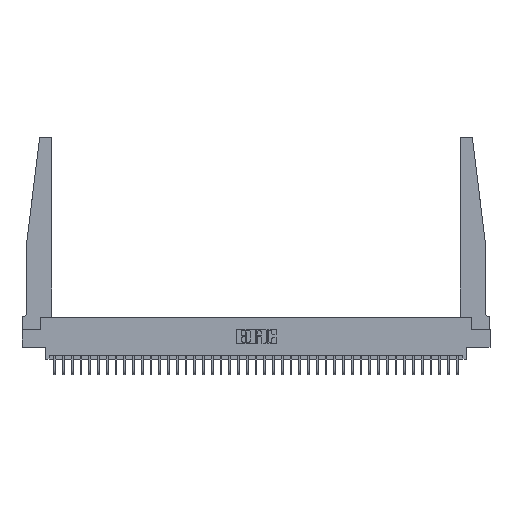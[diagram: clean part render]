
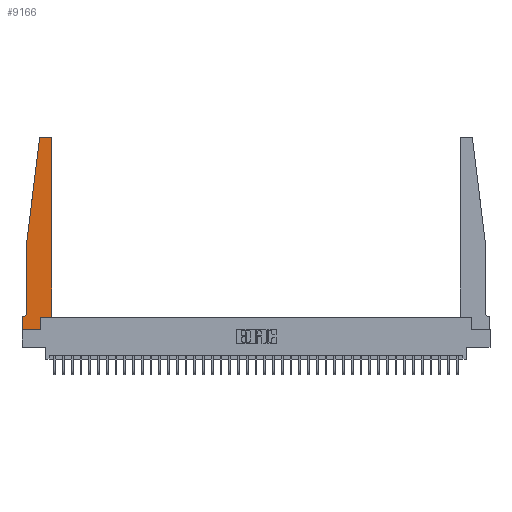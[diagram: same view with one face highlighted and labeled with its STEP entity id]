
A CAD part, top view. The second image highlights one B-rep face of the part: STEP entity #9166.
In plain terms, the highlighted planar face has unit normal (0, 0, 1).
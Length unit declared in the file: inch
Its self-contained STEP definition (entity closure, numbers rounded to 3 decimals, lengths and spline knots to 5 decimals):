
#387 = VERTEX_POINT ( 'NONE', #12092 ) ;
#510 = LINE ( 'NONE', #29118, #29665 ) ;
#821 = EDGE_CURVE ( 'NONE', #387, #16266, #21222, .T. ) ;
#1296 = DIRECTION ( 'NONE',  ( 0., 1., 0. ) ) ;
#1313 = EDGE_CURVE ( 'NONE', #24531, #387, #5923, .T. ) ;
#1544 = CARTESIAN_POINT ( 'NONE',  ( 0.25, 2.75, 0.37 ) ) ;
#2374 = VERTEX_POINT ( 'NONE', #12447 ) ;
#2948 = DIRECTION ( 'NONE',  ( -0.122, -0.992, 0. ) ) ;
#3323 = VECTOR ( 'NONE', #33705, 39.37008 ) ;
#3333 = CARTESIAN_POINT ( 'NONE',  ( 0.395, 2.72, 0.37 ) ) ;
#4560 = CARTESIAN_POINT ( 'NONE',  ( 0., 0., 0.37 ) ) ;
#5331 = ORIENTED_EDGE ( 'NONE', *, *, #36915, .T. ) ;
#5678 = VERTEX_POINT ( 'NONE', #19425 ) ;
#5923 = LINE ( 'NONE', #20399, #12283 ) ;
#6107 = CARTESIAN_POINT ( 'NONE',  ( 0.065, 1.25, 0.37 ) ) ;
#6130 = ORIENTED_EDGE ( 'NONE', *, *, #17333, .T. ) ;
#6385 = CARTESIAN_POINT ( 'NONE',  ( 0., 0., 0.37 ) ) ;
#6707 = ORIENTED_EDGE ( 'NONE', *, *, #17545, .T. ) ;
#7397 = ORIENTED_EDGE ( 'NONE', *, *, #15008, .T. ) ;
#8469 = LINE ( 'NONE', #19943, #34040 ) ;
#8623 = CARTESIAN_POINT ( 'NONE',  ( 0., 0., 0.37 ) ) ;
#8785 = DIRECTION ( 'NONE',  ( 1., 0., 0. ) ) ;
#9166 = ADVANCED_FACE ( 'NONE', ( #25499 ), #31516, .T. ) ;
#9380 = DIRECTION ( 'NONE',  ( 0., -1., 0. ) ) ;
#10082 = VERTEX_POINT ( 'NONE', #34422 ) ;
#10230 = EDGE_LOOP ( 'NONE', ( #35378, #15168, #11102, #34128, #7397, #25515, #29548, #6130, #5331, #6707, #31524, #20051 ) ) ;
#10434 = LINE ( 'NONE', #10616, #3323 ) ;
#10616 = CARTESIAN_POINT ( 'NONE',  ( 0.065, 0.1875, 0.37 ) ) ;
#11102 = ORIENTED_EDGE ( 'NONE', *, *, #15482, .T. ) ;
#11567 = CIRCLE ( 'NONE', #34339, 0.03 ) ;
#12092 = CARTESIAN_POINT ( 'NONE',  ( 0.425, 2.72, 0.37 ) ) ;
#12154 = CIRCLE ( 'NONE', #12748, 0.05 ) ;
#12283 = VECTOR ( 'NONE', #14789, 39.37008 ) ;
#12390 = DIRECTION ( 'NONE',  ( 0., 0., 1. ) ) ;
#12447 = CARTESIAN_POINT ( 'NONE',  ( 0.015, 0.1875, 0.37 ) ) ;
#12464 = VECTOR ( 'NONE', #35587, 39.37008 ) ;
#12748 = AXIS2_PLACEMENT_3D ( 'NONE', #20483, #17690, #29151 ) ;
#13088 = CARTESIAN_POINT ( 'NONE',  ( 0.27653, 2.75, 0.37 ) ) ;
#13323 = AXIS2_PLACEMENT_3D ( 'NONE', #28693, #31137, #14417 ) ;
#13412 = LINE ( 'NONE', #4560, #12464 ) ;
#14417 = DIRECTION ( 'NONE',  ( 1., 0., 0. ) ) ;
#14789 = DIRECTION ( 'NONE',  ( 0., 1., 0. ) ) ;
#14844 = DIRECTION ( 'NONE',  ( 0., -1., 0. ) ) ;
#15008 = EDGE_CURVE ( 'NONE', #25656, #2374, #12154, .T. ) ;
#15168 = ORIENTED_EDGE ( 'NONE', *, *, #31744, .T. ) ;
#15482 = EDGE_CURVE ( 'NONE', #10082, #15915, #34343, .T. ) ;
#15915 = VERTEX_POINT ( 'NONE', #6107 ) ;
#16266 = VERTEX_POINT ( 'NONE', #29349 ) ;
#16661 = CARTESIAN_POINT ( 'NONE',  ( 0., 0.1875, 0.37 ) ) ;
#16793 = DIRECTION ( 'NONE',  ( 1., 0., 0. ) ) ;
#17333 = EDGE_CURVE ( 'NONE', #31062, #22013, #13412, .T. ) ;
#17545 = EDGE_CURVE ( 'NONE', #5678, #24531, #8469, .T. ) ;
#17690 = DIRECTION ( 'NONE',  ( 0., 0., -1. ) ) ;
#18093 = EDGE_CURVE ( 'NONE', #36003, #31062, #25903, .T. ) ;
#19425 = CARTESIAN_POINT ( 'NONE',  ( 0.2605, 0.18, 0.37 ) ) ;
#19794 = CARTESIAN_POINT ( 'NONE',  ( 0.27653, 2.72, 0.37 ) ) ;
#19871 = CARTESIAN_POINT ( 'NONE',  ( 0.065, 0.2375, 0.37 ) ) ;
#19943 = CARTESIAN_POINT ( 'NONE',  ( 0.425, 0.18, 0.37 ) ) ;
#20051 = ORIENTED_EDGE ( 'NONE', *, *, #821, .T. ) ;
#20399 = CARTESIAN_POINT ( 'NONE',  ( 0.425, 0.18, 0.37 ) ) ;
#20483 = CARTESIAN_POINT ( 'NONE',  ( 0.015, 0.2375, 0.37 ) ) ;
#21222 = CIRCLE ( 'NONE', #33804, 0.03 ) ;
#22013 = VERTEX_POINT ( 'NONE', #32024 ) ;
#23125 = EDGE_CURVE ( 'NONE', #15915, #25656, #510, .T. ) ;
#24064 = LINE ( 'NONE', #27067, #31535 ) ;
#24531 = VERTEX_POINT ( 'NONE', #25127 ) ;
#24699 = EDGE_CURVE ( 'NONE', #2374, #36003, #10434, .T. ) ;
#25127 = CARTESIAN_POINT ( 'NONE',  ( 0.425, 0.18, 0.37 ) ) ;
#25350 = VECTOR ( 'NONE', #2948, 39.37008 ) ;
#25499 = FACE_OUTER_BOUND ( 'NONE', #10230, .T. ) ;
#25515 = ORIENTED_EDGE ( 'NONE', *, *, #24699, .T. ) ;
#25656 = VERTEX_POINT ( 'NONE', #19871 ) ;
#25903 = LINE ( 'NONE', #8623, #31068 ) ;
#27067 = CARTESIAN_POINT ( 'NONE',  ( 0.2605, 0.18, 0.37 ) ) ;
#27811 = VERTEX_POINT ( 'NONE', #13088 ) ;
#28194 = EDGE_CURVE ( 'NONE', #16266, #27811, #29955, .T. ) ;
#28693 = CARTESIAN_POINT ( 'NONE',  ( 0., 0.1875, 0.37 ) ) ;
#28717 = CARTESIAN_POINT ( 'NONE',  ( 0.065, 1.25, 0.37 ) ) ;
#29118 = CARTESIAN_POINT ( 'NONE',  ( 0.065, 1.25, 0.37 ) ) ;
#29151 = DIRECTION ( 'NONE',  ( -1., 0., 0. ) ) ;
#29349 = CARTESIAN_POINT ( 'NONE',  ( 0.395, 2.75, 0.37 ) ) ;
#29548 = ORIENTED_EDGE ( 'NONE', *, *, #18093, .T. ) ;
#29665 = VECTOR ( 'NONE', #14844, 39.37008 ) ;
#29955 = LINE ( 'NONE', #1544, #36502 ) ;
#31062 = VERTEX_POINT ( 'NONE', #6385 ) ;
#31068 = VECTOR ( 'NONE', #9380, 39.37008 ) ;
#31137 = DIRECTION ( 'NONE',  ( 0., 0., 1. ) ) ;
#31422 = DIRECTION ( 'NONE',  ( 1., 0., 0. ) ) ;
#31451 = DIRECTION ( 'NONE',  ( 0., 0., 1. ) ) ;
#31516 = PLANE ( 'NONE',  #13323 ) ;
#31524 = ORIENTED_EDGE ( 'NONE', *, *, #1313, .T. ) ;
#31535 = VECTOR ( 'NONE', #1296, 39.37008 ) ;
#31744 = EDGE_CURVE ( 'NONE', #27811, #10082, #11567, .T. ) ;
#32024 = CARTESIAN_POINT ( 'NONE',  ( 0.2605, 0., 0.37 ) ) ;
#32777 = DIRECTION ( 'NONE',  ( -1., 0., 0. ) ) ;
#33705 = DIRECTION ( 'NONE',  ( -1., 0., 0. ) ) ;
#33804 = AXIS2_PLACEMENT_3D ( 'NONE', #3333, #12390, #8785 ) ;
#34040 = VECTOR ( 'NONE', #31422, 39.37008 ) ;
#34128 = ORIENTED_EDGE ( 'NONE', *, *, #23125, .T. ) ;
#34339 = AXIS2_PLACEMENT_3D ( 'NONE', #19794, #31451, #16793 ) ;
#34343 = LINE ( 'NONE', #28717, #25350 ) ;
#34422 = CARTESIAN_POINT ( 'NONE',  ( 0.24675, 2.72367, 0.37 ) ) ;
#35378 = ORIENTED_EDGE ( 'NONE', *, *, #28194, .T. ) ;
#35587 = DIRECTION ( 'NONE',  ( 1., 0., 0. ) ) ;
#36003 = VERTEX_POINT ( 'NONE', #16661 ) ;
#36502 = VECTOR ( 'NONE', #32777, 39.37008 ) ;
#36915 = EDGE_CURVE ( 'NONE', #22013, #5678, #24064, .T. ) ;
